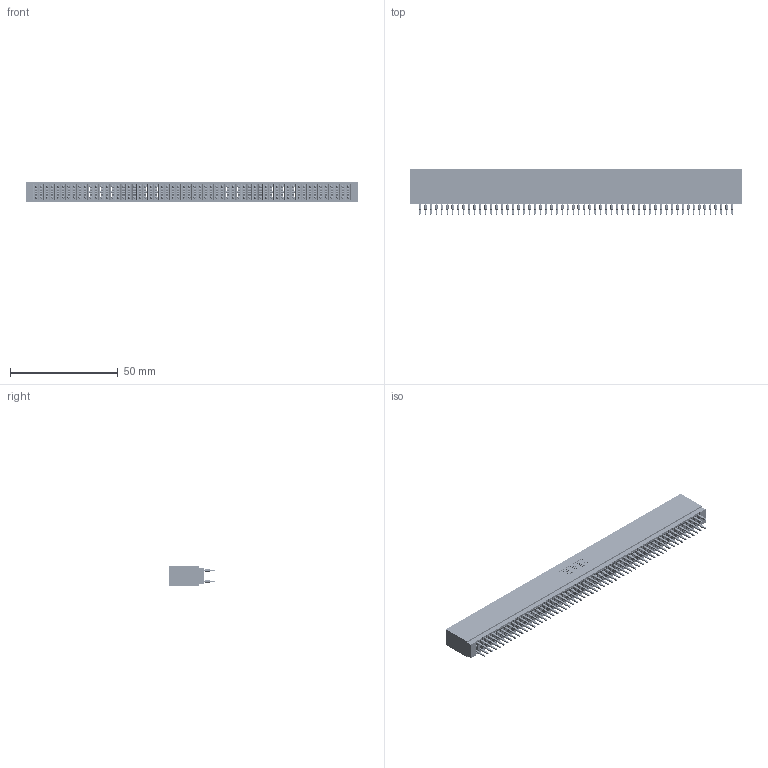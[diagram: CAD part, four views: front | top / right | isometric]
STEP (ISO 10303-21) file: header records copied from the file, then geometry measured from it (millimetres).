
FILE_DESCRIPTION (( 'STEP AP203' ), '1' );
FILE_NAME ('745-116-560-201.STEP', '2026-02-27T01:03:03', ( '' ), ( '' ), 'SwSTEP 2.0', 'SolidWorks 2023', '' );
FILE_SCHEMA (( 'CONFIG_CONTROL_DESIGN' ));
Products named in the file (3): 745-292-001_560; 745-116-560-201; 745 Part_Insulator Option - 01
Assembly tree (117 placements, depth 2):
  745-116-560-201
    745 Part_Insulator Option - 01
    745-292-001_560  x116
Bounding box: 153.92 x 21.22 x 8.89 mm (x, y, z)
Volume: 14194.8 mm3; surface area: 31056.5 mm2
Topology: 117 solids, 117 shells, 11521 faces, 31520 edges, 20008 vertices
Faces by surface type: plane 5971, cylinder 2534, bspline 2320, torus 696
Entity records: 95783 total; most frequent: CARTESIAN_POINT 17113, ORIENTED_EDGE 16580, DIRECTION 14474, EDGE_CURVE 8290, LINE 7752, VECTOR 7752, VERTEX_POINT 5288, AXIS2_PLACEMENT_3D 3361
